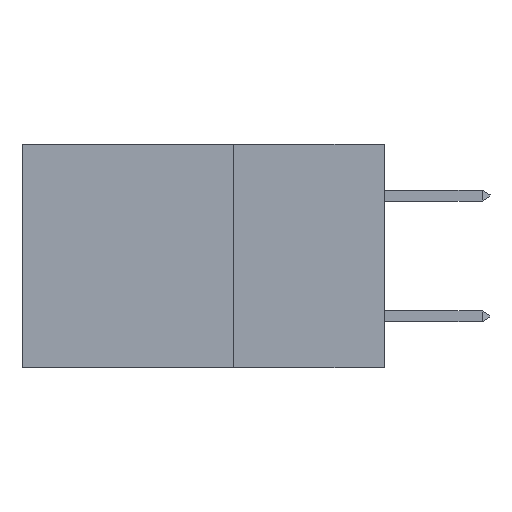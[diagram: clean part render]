
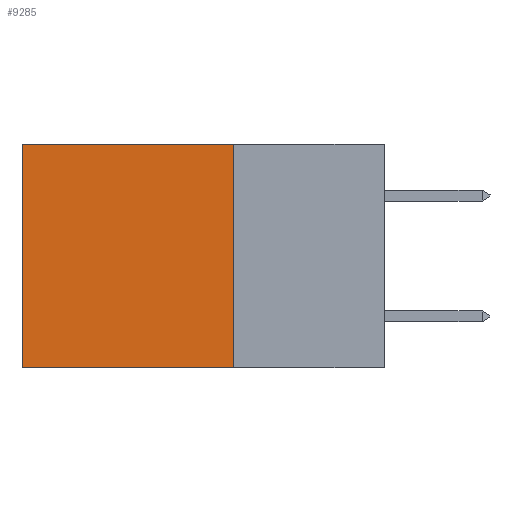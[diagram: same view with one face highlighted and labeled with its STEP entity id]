
A CAD part, left-side view. The second image highlights one B-rep face of the part: STEP entity #9285.
In plain terms, the highlighted planar face has unit normal (-1, 0, 0).
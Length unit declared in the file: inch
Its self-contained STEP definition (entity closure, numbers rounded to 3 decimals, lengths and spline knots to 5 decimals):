
#2212 = DIRECTION ( 'NONE',  ( 0., 0., -1. ) ) ;
#2372 = ORIENTED_EDGE ( 'NONE', *, *, #23796, .T. ) ;
#3418 = CARTESIAN_POINT ( 'NONE',  ( 0.2875, 0.25, -0.37 ) ) ;
#4170 = CARTESIAN_POINT ( 'NONE',  ( 0.2875, 0.25, 0. ) ) ;
#4207 = VECTOR ( 'NONE', #2212, 39.37008 ) ;
#4378 = DIRECTION ( 'NONE',  ( 0., 0., -1. ) ) ;
#7353 = LINE ( 'NONE', #28228, #26605 ) ;
#8482 = CARTESIAN_POINT ( 'NONE',  ( 0.2875, 0.25, 0. ) ) ;
#9260 = EDGE_CURVE ( 'NONE', #28220, #25125, #23523, .T. ) ;
#9285 = ADVANCED_FACE ( 'NONE', ( #33060 ), #27614, .F. ) ;
#10002 = VERTEX_POINT ( 'NONE', #30419 ) ;
#10035 = CARTESIAN_POINT ( 'NONE',  ( 0.2875, 0.6, 0. ) ) ;
#14366 = AXIS2_PLACEMENT_3D ( 'NONE', #8482, #31956, #4378 ) ;
#16140 = DIRECTION ( 'NONE',  ( 0., 1., 0. ) ) ;
#16347 = ORIENTED_EDGE ( 'NONE', *, *, #26581, .F. ) ;
#16417 = VECTOR ( 'NONE', #25317, 39.37008 ) ;
#16846 = VERTEX_POINT ( 'NONE', #3418 ) ;
#19699 = LINE ( 'NONE', #28000, #16417 ) ;
#20943 = DIRECTION ( 'NONE',  ( 0., 1., 0. ) ) ;
#21910 = VECTOR ( 'NONE', #16140, 39.37008 ) ;
#22469 = EDGE_LOOP ( 'NONE', ( #2372, #26474, #16347, #31632 ) ) ;
#23523 = LINE ( 'NONE', #32130, #21910 ) ;
#23796 = EDGE_CURVE ( 'NONE', #25125, #10002, #25028, .T. ) ;
#25028 = LINE ( 'NONE', #25359, #4207 ) ;
#25125 = VERTEX_POINT ( 'NONE', #10035 ) ;
#25317 = DIRECTION ( 'NONE',  ( 0., 0., -1. ) ) ;
#25359 = CARTESIAN_POINT ( 'NONE',  ( 0.2875, 0.6, 0. ) ) ;
#26474 = ORIENTED_EDGE ( 'NONE', *, *, #26629, .F. ) ;
#26581 = EDGE_CURVE ( 'NONE', #28220, #16846, #19699, .T. ) ;
#26605 = VECTOR ( 'NONE', #20943, 39.37008 ) ;
#26629 = EDGE_CURVE ( 'NONE', #16846, #10002, #7353, .T. ) ;
#27614 = PLANE ( 'NONE',  #14366 ) ;
#28000 = CARTESIAN_POINT ( 'NONE',  ( 0.2875, 0.25, 0. ) ) ;
#28220 = VERTEX_POINT ( 'NONE', #4170 ) ;
#28228 = CARTESIAN_POINT ( 'NONE',  ( 0.2875, 0.25, -0.37 ) ) ;
#30419 = CARTESIAN_POINT ( 'NONE',  ( 0.2875, 0.6, -0.37 ) ) ;
#31632 = ORIENTED_EDGE ( 'NONE', *, *, #9260, .T. ) ;
#31956 = DIRECTION ( 'NONE',  ( 1., 0., 0. ) ) ;
#32130 = CARTESIAN_POINT ( 'NONE',  ( 0.2875, 0.25, 0. ) ) ;
#33060 = FACE_OUTER_BOUND ( 'NONE', #22469, .T. ) ;
